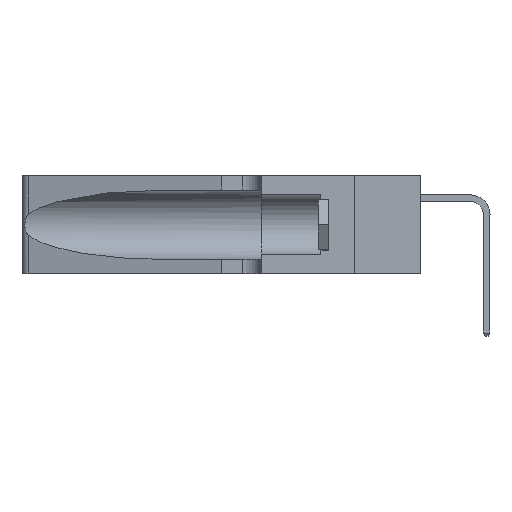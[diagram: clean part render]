
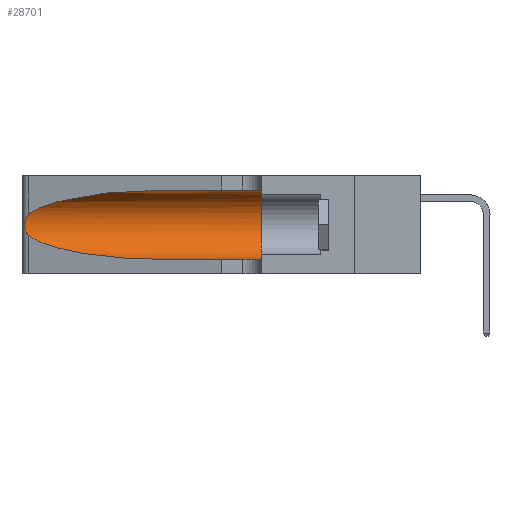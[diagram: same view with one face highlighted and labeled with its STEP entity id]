
A CAD part, left-side view. The second image highlights one B-rep face of the part: STEP entity #28701.
In plain terms, the highlighted cylindrical face has radius 3.308 mm (diameter 6.617 mm), a partial arc.
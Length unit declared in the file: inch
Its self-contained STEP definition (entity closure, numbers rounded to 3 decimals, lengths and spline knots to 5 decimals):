
#55 = CARTESIAN_POINT ( 'NONE',  ( 0.18966, 0.96281, 0.05475 ) ) ;
#599 = CARTESIAN_POINT ( 'NONE',  ( 0.1305, 0.72297, 0.05475 ) ) ;
#690 = CARTESIAN_POINT ( 'NONE',  ( 0.26017, 1.23833, 0.17102 ) ) ;
#824 = CARTESIAN_POINT ( 'NONE',  ( 0.2373, 1.15595, 0.28018 ) ) ;
#2399 = VERTEX_POINT ( 'NONE', #599 ) ;
#2639 = CARTESIAN_POINT ( 'NONE',  ( 0.25487, 1.22718, 0.14631 ) ) ;
#2648 = CARTESIAN_POINT ( 'NONE',  ( 0.1305, 1.61858, 0.185 ) ) ;
#2760 = ORIENTED_EDGE ( 'NONE', *, *, #23953, .T. ) ;
#3184 = CARTESIAN_POINT ( 'NONE',  ( 0.25789, 1.23486, 0.15765 ) ) ;
#3591 = VERTEX_POINT ( 'NONE', #2639 ) ;
#4539 = ORIENTED_EDGE ( 'NONE', *, *, #29695, .F. ) ;
#4549 = CIRCLE ( 'NONE', #28543, 0.13025 ) ;
#5539 = CARTESIAN_POINT ( 'NONE',  ( 0.1305, 0.35, 0.31525 ) ) ;
#5582 = CARTESIAN_POINT ( 'NONE',  ( 0.1305, 0.35, 0.185 ) ) ;
#5711 = CARTESIAN_POINT ( 'NONE',  ( 0.25555, 1.22993, 0.14849 ) ) ;
#6581 =( BOUNDED_CURVE ( )  B_SPLINE_CURVE ( 3, ( #27210, #10000, #55, #17470 ),
 .UNSPECIFIED., .F., .T. ) 
 B_SPLINE_CURVE_WITH_KNOTS ( ( 4, 4 ),
 ( 3.44316, 4.71239 ),
 .UNSPECIFIED. ) 
 CURVE ( )  GEOMETRIC_REPRESENTATION_ITEM ( )  RATIONAL_B_SPLINE_CURVE ( ( 1., 0.87, 0.87, 1. ) ) 
 REPRESENTATION_ITEM ( '' )  );
#7944 = CARTESIAN_POINT ( 'NONE',  ( 0.1305, 1.61858, 0.05475 ) ) ;
#8096 = DIRECTION ( 'NONE',  ( 0., 0., 1. ) ) ;
#8108 = CARTESIAN_POINT ( 'NONE',  ( 0.25487, 1.22718, 0.22369 ) ) ;
#9302 = CARTESIAN_POINT ( 'NONE',  ( 0.25487, 1.22718, 0.22369 ) ) ;
#10000 = CARTESIAN_POINT ( 'NONE',  ( 0.2373, 1.15595, 0.08982 ) ) ;
#10006 = B_SPLINE_CURVE_WITH_KNOTS ( 'NONE', 3,
 ( #8108, #22883, #25324, #10606, #27824, #13128, #30275, #15615, #690, #18081, #3184, #20535, #5711, #22987 ),
 .UNSPECIFIED., .F., .F.,
 ( 4, 2, 2, 2, 2, 2, 4 ),
 ( 0., 0.00027, 0.00053, 0.00107, 0.0016, 0.00187, 0.00214 ),
 .UNSPECIFIED. ) ;
#10606 = CARTESIAN_POINT ( 'NONE',  ( 0.25787, 1.23484, 0.2124 ) ) ;
#10752 = CARTESIAN_POINT ( 'NONE',  ( 0.18966, 0.96281, 0.31525 ) ) ;
#12583 = DIRECTION ( 'NONE',  ( 0., 0., -1. ) ) ;
#13128 = CARTESIAN_POINT ( 'NONE',  ( 0.26018, 1.23835, 0.19895 ) ) ;
#13945 = DIRECTION ( 'NONE',  ( 0., -1., 0. ) ) ;
#15185 = DIRECTION ( 'NONE',  ( 0., -1., 0. ) ) ;
#15326 = CYLINDRICAL_SURFACE ( 'NONE', #18332, 0.13025 ) ;
#15615 = CARTESIAN_POINT ( 'NONE',  ( 0.26075, 1.23896, 0.178 ) ) ;
#15961 =( BOUNDED_CURVE ( )  B_SPLINE_CURVE ( 3, ( #30417, #10752, #824, #18218 ),
 .UNSPECIFIED., .F., .F. ) 
 B_SPLINE_CURVE_WITH_KNOTS ( ( 4, 4 ),
 ( 1.5708, 2.84003 ),
 .UNSPECIFIED. ) 
 CURVE ( )  GEOMETRIC_REPRESENTATION_ITEM ( )  RATIONAL_B_SPLINE_CURVE ( ( 1., 0.87, 0.87, 1. ) ) 
 REPRESENTATION_ITEM ( '' )  );
#16883 = EDGE_LOOP ( 'NONE', ( #17180, #19147, #2760, #26555, #30462, #4539 ) ) ;
#17180 = ORIENTED_EDGE ( 'NONE', *, *, #28199, .T. ) ;
#17470 = CARTESIAN_POINT ( 'NONE',  ( 0.1305, 0.72297, 0.05475 ) ) ;
#17929 = LINE ( 'NONE', #31079, #23646 ) ;
#18081 = CARTESIAN_POINT ( 'NONE',  ( 0.25856, 1.23593, 0.16098 ) ) ;
#18218 = CARTESIAN_POINT ( 'NONE',  ( 0.25487, 1.22718, 0.22369 ) ) ;
#18332 = AXIS2_PLACEMENT_3D ( 'NONE', #2648, #15185, #12583 ) ;
#18826 = CARTESIAN_POINT ( 'NONE',  ( 0.1305, 0.35, 0.05475 ) ) ;
#19147 = ORIENTED_EDGE ( 'NONE', *, *, #20830, .T. ) ;
#19690 = EDGE_CURVE ( 'NONE', #2399, #21023, #23284, .T. ) ;
#20535 = CARTESIAN_POINT ( 'NONE',  ( 0.25639, 1.23186, 0.15144 ) ) ;
#20830 = EDGE_CURVE ( 'NONE', #30687, #3591, #10006, .T. ) ;
#21023 = VERTEX_POINT ( 'NONE', #18826 ) ;
#21163 = VERTEX_POINT ( 'NONE', #25951 ) ;
#22604 = FACE_OUTER_BOUND ( 'NONE', #16883, .T. ) ;
#22752 = DIRECTION ( 'NONE',  ( 0., -1., 0. ) ) ;
#22874 = DIRECTION ( 'NONE',  ( 0., 1., 0. ) ) ;
#22883 = CARTESIAN_POINT ( 'NONE',  ( 0.25555, 1.22994, 0.2215 ) ) ;
#22987 = CARTESIAN_POINT ( 'NONE',  ( 0.25487, 1.22718, 0.14631 ) ) ;
#23284 = LINE ( 'NONE', #7944, #30594 ) ;
#23646 = VECTOR ( 'NONE', #13945, 39.37008 ) ;
#23953 = EDGE_CURVE ( 'NONE', #3591, #2399, #6581, .T. ) ;
#24717 = VERTEX_POINT ( 'NONE', #5539 ) ;
#25324 = CARTESIAN_POINT ( 'NONE',  ( 0.25639, 1.23184, 0.21858 ) ) ;
#25951 = CARTESIAN_POINT ( 'NONE',  ( 0.1305, 0.72297, 0.31525 ) ) ;
#26555 = ORIENTED_EDGE ( 'NONE', *, *, #19690, .T. ) ;
#26988 = EDGE_CURVE ( 'NONE', #24717, #21023, #4549, .T. ) ;
#27210 = CARTESIAN_POINT ( 'NONE',  ( 0.25487, 1.22718, 0.14631 ) ) ;
#27824 = CARTESIAN_POINT ( 'NONE',  ( 0.25854, 1.2359, 0.20912 ) ) ;
#28199 = EDGE_CURVE ( 'NONE', #21163, #30687, #15961, .T. ) ;
#28543 = AXIS2_PLACEMENT_3D ( 'NONE', #5582, #22874, #8096 ) ;
#28701 = ADVANCED_FACE ( 'NONE', ( #22604 ), #15326, .F. ) ;
#29695 = EDGE_CURVE ( 'NONE', #21163, #24717, #17929, .T. ) ;
#30275 = CARTESIAN_POINT ( 'NONE',  ( 0.26075, 1.23896, 0.19203 ) ) ;
#30417 = CARTESIAN_POINT ( 'NONE',  ( 0.1305, 0.72297, 0.31525 ) ) ;
#30462 = ORIENTED_EDGE ( 'NONE', *, *, #26988, .F. ) ;
#30594 = VECTOR ( 'NONE', #22752, 39.37008 ) ;
#30687 = VERTEX_POINT ( 'NONE', #9302 ) ;
#31079 = CARTESIAN_POINT ( 'NONE',  ( 0.1305, 1.61858, 0.31525 ) ) ;
